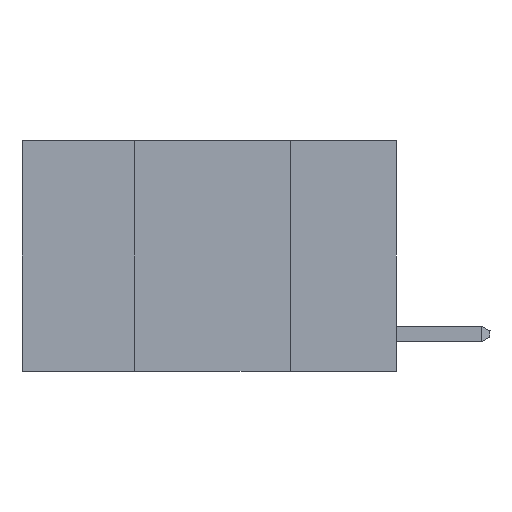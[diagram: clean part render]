
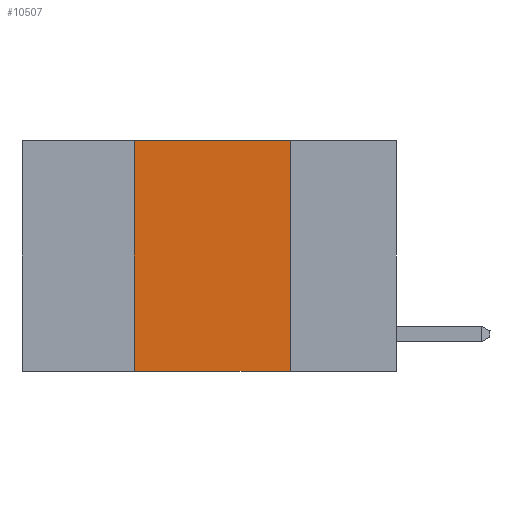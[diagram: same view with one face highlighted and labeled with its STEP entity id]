
A CAD part, left-side view. The second image highlights one B-rep face of the part: STEP entity #10507.
In plain terms, the highlighted planar face has unit normal (-1, 0, 0).
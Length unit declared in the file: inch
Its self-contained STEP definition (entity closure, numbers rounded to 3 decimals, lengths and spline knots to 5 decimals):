
#275 = EDGE_CURVE ( 'NONE', #5927, #9351, #9360, .T. ) ;
#298 = ORIENTED_EDGE ( 'NONE', *, *, #11089, .T. ) ;
#354 = ORIENTED_EDGE ( 'NONE', *, *, #1086, .F. ) ;
#619 = LINE ( 'NONE', #9256, #9362 ) ;
#1086 = EDGE_CURVE ( 'NONE', #2706, #4143, #5278, .T. ) ;
#1292 = AXIS2_PLACEMENT_3D ( 'NONE', #4268, #4234, #8603 ) ;
#1391 = ORIENTED_EDGE ( 'NONE', *, *, #8934, .F. ) ;
#2378 = DIRECTION ( 'NONE',  ( 0., -1., 0. ) ) ;
#2706 = VERTEX_POINT ( 'NONE', #9799 ) ;
#2846 = CARTESIAN_POINT ( 'NONE',  ( 0., 0.42, 0. ) ) ;
#3019 = CARTESIAN_POINT ( 'NONE',  ( 0., 0.6, -0.37 ) ) ;
#3879 = DIRECTION ( 'NONE',  ( 0., -1., 0. ) ) ;
#4143 = VERTEX_POINT ( 'NONE', #2846 ) ;
#4234 = DIRECTION ( 'NONE',  ( 1., 0., 0. ) ) ;
#4268 = CARTESIAN_POINT ( 'NONE',  ( 0., 0.6, 0. ) ) ;
#4342 = LINE ( 'NONE', #3019, #5943 ) ;
#4767 = FACE_OUTER_BOUND ( 'NONE', #5595, .T. ) ;
#4839 = ORIENTED_EDGE ( 'NONE', *, *, #275, .F. ) ;
#4932 = CARTESIAN_POINT ( 'NONE',  ( 0., 0.17, -0.37 ) ) ;
#5278 = LINE ( 'NONE', #9330, #9314 ) ;
#5480 = CARTESIAN_POINT ( 'NONE',  ( 0., 0.17, 0. ) ) ;
#5595 = EDGE_LOOP ( 'NONE', ( #4839, #1391, #354, #298 ) ) ;
#5927 = VERTEX_POINT ( 'NONE', #5480 ) ;
#5943 = VECTOR ( 'NONE', #3879, 39.37008 ) ;
#8603 = DIRECTION ( 'NONE',  ( 0., 0., -1. ) ) ;
#8934 = EDGE_CURVE ( 'NONE', #4143, #5927, #619, .T. ) ;
#9256 = CARTESIAN_POINT ( 'NONE',  ( 0., 0.6, 0. ) ) ;
#9266 = DIRECTION ( 'NONE',  ( 0., 0., 1. ) ) ;
#9314 = VECTOR ( 'NONE', #9266, 39.37008 ) ;
#9330 = CARTESIAN_POINT ( 'NONE',  ( 0., 0.42, 0. ) ) ;
#9351 = VERTEX_POINT ( 'NONE', #4932 ) ;
#9360 = LINE ( 'NONE', #9505, #9602 ) ;
#9362 = VECTOR ( 'NONE', #2378, 39.37008 ) ;
#9505 = CARTESIAN_POINT ( 'NONE',  ( 0., 0.17, 0. ) ) ;
#9539 = DIRECTION ( 'NONE',  ( 0., 0., -1. ) ) ;
#9602 = VECTOR ( 'NONE', #9539, 39.37008 ) ;
#9799 = CARTESIAN_POINT ( 'NONE',  ( 0., 0.42, -0.37 ) ) ;
#10300 = PLANE ( 'NONE',  #1292 ) ;
#10507 = ADVANCED_FACE ( 'NONE', ( #4767 ), #10300, .F. ) ;
#11089 = EDGE_CURVE ( 'NONE', #2706, #9351, #4342, .T. ) ;
